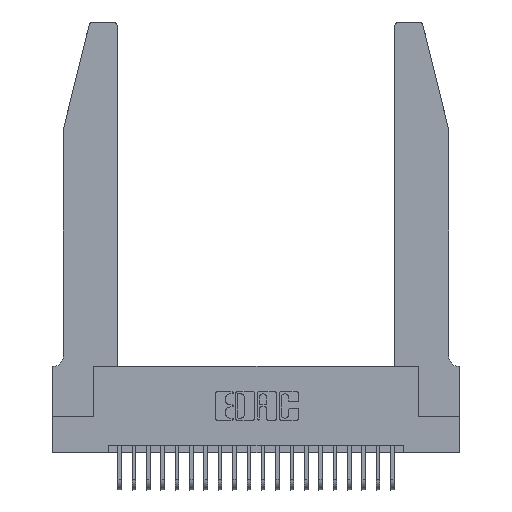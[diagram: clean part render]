
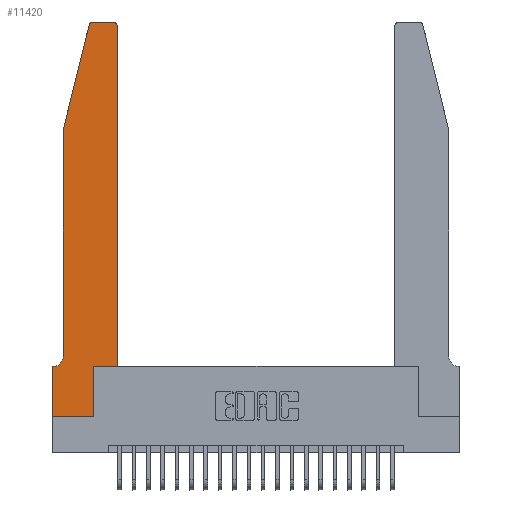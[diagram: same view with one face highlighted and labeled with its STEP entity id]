
A CAD part, top view. The second image highlights one B-rep face of the part: STEP entity #11420.
In plain terms, the highlighted planar face has unit normal (0, 0, 1).
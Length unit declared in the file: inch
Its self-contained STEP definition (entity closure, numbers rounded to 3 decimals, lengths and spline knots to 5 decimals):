
#54 = AXIS2_PLACEMENT_3D ( 'NONE', #12730, #2009, #14460 ) ;
#113 = ORIENTED_EDGE ( 'NONE', *, *, #12898, .T. ) ;
#268 = DIRECTION ( 'NONE',  ( -1., 0., 0. ) ) ;
#366 = ORIENTED_EDGE ( 'NONE', *, *, #4739, .T. ) ;
#371 = EDGE_LOOP ( 'NONE', ( #3815, #16749, #12206, #8585, #12159, #5751, #928, #366, #4051, #2353, #20517, #113 ) ) ;
#389 = DIRECTION ( 'NONE',  ( -1., 0., 0. ) ) ;
#853 = VERTEX_POINT ( 'NONE', #16034 ) ;
#928 = ORIENTED_EDGE ( 'NONE', *, *, #2285, .T. ) ;
#1128 = VERTEX_POINT ( 'NONE', #13368 ) ;
#1559 = CARTESIAN_POINT ( 'NONE',  ( 0.4505, 0.35, 0.37 ) ) ;
#1641 = DIRECTION ( 'NONE',  ( 0., 1., 0. ) ) ;
#2009 = DIRECTION ( 'NONE',  ( 0., 0., 1. ) ) ;
#2139 = EDGE_CURVE ( 'NONE', #22439, #11252, #6534, .T. ) ;
#2285 = EDGE_CURVE ( 'NONE', #6539, #8266, #8514, .T. ) ;
#2353 = ORIENTED_EDGE ( 'NONE', *, *, #21929, .T. ) ;
#2773 = LINE ( 'NONE', #11051, #15772 ) ;
#2803 = EDGE_CURVE ( 'NONE', #853, #21095, #3099, .T. ) ;
#2908 = VERTEX_POINT ( 'NONE', #11618 ) ;
#3099 = LINE ( 'NONE', #19911, #17146 ) ;
#3279 = VECTOR ( 'NONE', #3380, 39.37008 ) ;
#3380 = DIRECTION ( 'NONE',  ( 1., 0., 0. ) ) ;
#3683 = VERTEX_POINT ( 'NONE', #7841 ) ;
#3698 = VECTOR ( 'NONE', #20321, 39.37008 ) ;
#3815 = ORIENTED_EDGE ( 'NONE', *, *, #20223, .T. ) ;
#4051 = ORIENTED_EDGE ( 'NONE', *, *, #2139, .T. ) ;
#4215 = CARTESIAN_POINT ( 'NONE',  ( 0.2865, 0.35, 0.37 ) ) ;
#4650 = VERTEX_POINT ( 'NONE', #10890 ) ;
#4671 = EDGE_CURVE ( 'NONE', #5515, #1128, #4725, .T. ) ;
#4725 = CIRCLE ( 'NONE', #54, 0.03 ) ;
#4739 = EDGE_CURVE ( 'NONE', #8266, #22439, #7271, .T. ) ;
#5366 = EDGE_CURVE ( 'NONE', #4650, #6539, #9550, .T. ) ;
#5515 = VERTEX_POINT ( 'NONE', #16714 ) ;
#5751 = ORIENTED_EDGE ( 'NONE', *, *, #5366, .T. ) ;
#5815 = EDGE_CURVE ( 'NONE', #2908, #3683, #14152, .T. ) ;
#5828 = DIRECTION ( 'NONE',  ( 0., 0., 1. ) ) ;
#5973 = VECTOR ( 'NONE', #9594, 39.37008 ) ;
#6441 = CIRCLE ( 'NONE', #18528, 0.03 ) ;
#6534 = LINE ( 'NONE', #7783, #5973 ) ;
#6539 = VERTEX_POINT ( 'NONE', #9917 ) ;
#6952 = EDGE_CURVE ( 'NONE', #21095, #4650, #18379, .T. ) ;
#7271 = LINE ( 'NONE', #9379, #20620 ) ;
#7753 = DIRECTION ( 'NONE',  ( 0., -1., 0. ) ) ;
#7783 = CARTESIAN_POINT ( 'NONE',  ( 0.2865, 0.35, 0.37 ) ) ;
#7841 = CARTESIAN_POINT ( 'NONE',  ( 0.4505, 2.72, 0.37 ) ) ;
#8113 = LINE ( 'NONE', #1559, #3279 ) ;
#8266 = VERTEX_POINT ( 'NONE', #18305 ) ;
#8460 = FACE_OUTER_BOUND ( 'NONE', #371, .T. ) ;
#8514 = LINE ( 'NONE', #18482, #3698 ) ;
#8585 = ORIENTED_EDGE ( 'NONE', *, *, #2803, .T. ) ;
#8811 = CARTESIAN_POINT ( 'NONE',  ( 0., 0.35, 0.37 ) ) ;
#9379 = CARTESIAN_POINT ( 'NONE',  ( 0., 0., 0.37 ) ) ;
#9550 = LINE ( 'NONE', #21550, #22820 ) ;
#9594 = DIRECTION ( 'NONE',  ( 0., 1., 0. ) ) ;
#9731 = LINE ( 'NONE', #11989, #18385 ) ;
#9917 = CARTESIAN_POINT ( 'NONE',  ( 0., 0.35, 0.37 ) ) ;
#10565 = DIRECTION ( 'NONE',  ( 1., 0., 0. ) ) ;
#10593 = CARTESIAN_POINT ( 'NONE',  ( 0.4505, 0.35, 0.37 ) ) ;
#10890 = CARTESIAN_POINT ( 'NONE',  ( 0.0055, 0.35, 0.37 ) ) ;
#10992 = AXIS2_PLACEMENT_3D ( 'NONE', #8811, #20950, #10565 ) ;
#11039 = DIRECTION ( 'NONE',  ( 0., 0., -1. ) ) ;
#11051 = CARTESIAN_POINT ( 'NONE',  ( 0.0755, 2., 0.37 ) ) ;
#11110 = DIRECTION ( 'NONE',  ( 1., 0., 0. ) ) ;
#11252 = VERTEX_POINT ( 'NONE', #4215 ) ;
#11420 = ADVANCED_FACE ( 'NONE', ( #8460 ), #14017, .T. ) ;
#11618 = CARTESIAN_POINT ( 'NONE',  ( 0.4505, 0.35, 0.37 ) ) ;
#11989 = CARTESIAN_POINT ( 'NONE',  ( 0.2605, 2.75, 0.37 ) ) ;
#12159 = ORIENTED_EDGE ( 'NONE', *, *, #6952, .T. ) ;
#12206 = ORIENTED_EDGE ( 'NONE', *, *, #12893, .T. ) ;
#12730 = CARTESIAN_POINT ( 'NONE',  ( 0.284, 2.72, 0.37 ) ) ;
#12893 = EDGE_CURVE ( 'NONE', #1128, #853, #2773, .T. ) ;
#12898 = EDGE_CURVE ( 'NONE', #3683, #13951, #6441, .T. ) ;
#13368 = CARTESIAN_POINT ( 'NONE',  ( 0.25487, 2.72718, 0.37 ) ) ;
#13951 = VERTEX_POINT ( 'NONE', #21158 ) ;
#14017 = PLANE ( 'NONE',  #10992 ) ;
#14152 = LINE ( 'NONE', #10593, #19244 ) ;
#14460 = DIRECTION ( 'NONE',  ( 1., 0., 0. ) ) ;
#15772 = VECTOR ( 'NONE', #17987, 39.37008 ) ;
#16034 = CARTESIAN_POINT ( 'NONE',  ( 0.0755, 2., 0.37 ) ) ;
#16313 = CARTESIAN_POINT ( 'NONE',  ( 0.4205, 2.72, 0.37 ) ) ;
#16411 = AXIS2_PLACEMENT_3D ( 'NONE', #21424, #11039, #268 ) ;
#16714 = CARTESIAN_POINT ( 'NONE',  ( 0.284, 2.75, 0.37 ) ) ;
#16749 = ORIENTED_EDGE ( 'NONE', *, *, #4671, .T. ) ;
#17146 = VECTOR ( 'NONE', #7753, 39.37008 ) ;
#17987 = DIRECTION ( 'NONE',  ( -0.239, -0.971, 0. ) ) ;
#18067 = DIRECTION ( 'NONE',  ( 1., 0., 0. ) ) ;
#18305 = CARTESIAN_POINT ( 'NONE',  ( 0., 0., 0.37 ) ) ;
#18379 = CIRCLE ( 'NONE', #16411, 0.07 ) ;
#18385 = VECTOR ( 'NONE', #18817, 39.37008 ) ;
#18482 = CARTESIAN_POINT ( 'NONE',  ( 0., 0., 0.37 ) ) ;
#18528 = AXIS2_PLACEMENT_3D ( 'NONE', #16313, #5828, #18067 ) ;
#18799 = CARTESIAN_POINT ( 'NONE',  ( 0.2865, 0., 0.37 ) ) ;
#18817 = DIRECTION ( 'NONE',  ( -1., 0., 0. ) ) ;
#19244 = VECTOR ( 'NONE', #1641, 39.37008 ) ;
#19911 = CARTESIAN_POINT ( 'NONE',  ( 0.0755, 2., 0.37 ) ) ;
#20223 = EDGE_CURVE ( 'NONE', #13951, #5515, #9731, .T. ) ;
#20255 = CARTESIAN_POINT ( 'NONE',  ( 0.0755, 0.42, 0.37 ) ) ;
#20321 = DIRECTION ( 'NONE',  ( 0., -1., 0. ) ) ;
#20517 = ORIENTED_EDGE ( 'NONE', *, *, #5815, .T. ) ;
#20620 = VECTOR ( 'NONE', #11110, 39.37008 ) ;
#20950 = DIRECTION ( 'NONE',  ( 0., 0., 1. ) ) ;
#21095 = VERTEX_POINT ( 'NONE', #20255 ) ;
#21158 = CARTESIAN_POINT ( 'NONE',  ( 0.4205, 2.75, 0.37 ) ) ;
#21424 = CARTESIAN_POINT ( 'NONE',  ( 0.0055, 0.42, 0.37 ) ) ;
#21550 = CARTESIAN_POINT ( 'NONE',  ( 0.0755, 0.35, 0.37 ) ) ;
#21929 = EDGE_CURVE ( 'NONE', #11252, #2908, #8113, .T. ) ;
#22439 = VERTEX_POINT ( 'NONE', #18799 ) ;
#22820 = VECTOR ( 'NONE', #389, 39.37008 ) ;
